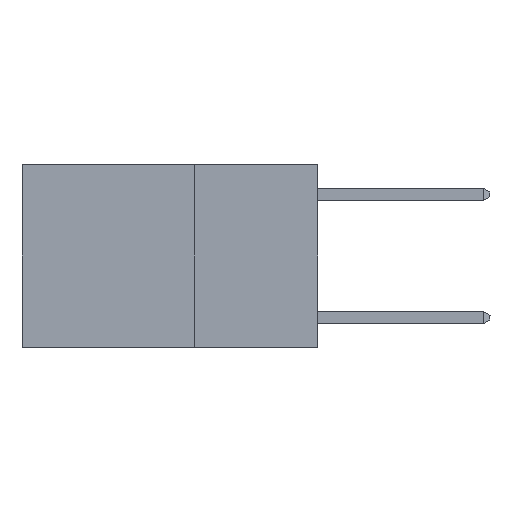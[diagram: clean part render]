
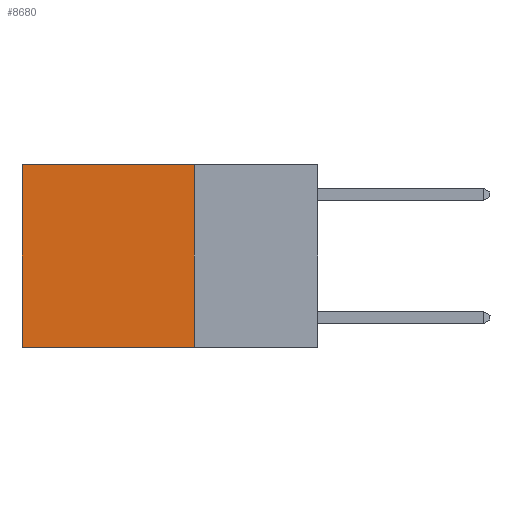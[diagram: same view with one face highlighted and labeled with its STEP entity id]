
A CAD part, left-side view. The second image highlights one B-rep face of the part: STEP entity #8680.
In plain terms, the highlighted planar face has unit normal (-1, 0, 0).
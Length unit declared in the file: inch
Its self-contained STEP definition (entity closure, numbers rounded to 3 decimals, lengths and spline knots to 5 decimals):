
#239 = LINE ( 'NONE', #921, #6667 ) ;
#490 = DIRECTION ( 'NONE',  ( 0., 0., -1. ) ) ;
#635 = AXIS2_PLACEMENT_3D ( 'NONE', #1219, #5118, #490 ) ;
#921 = CARTESIAN_POINT ( 'NONE',  ( 0.2625, 0.25, -0.37 ) ) ;
#1219 = CARTESIAN_POINT ( 'NONE',  ( 0.2625, 0.25, 0. ) ) ;
#1326 = DIRECTION ( 'NONE',  ( 0., 0., -1. ) ) ;
#1736 = CARTESIAN_POINT ( 'NONE',  ( 0.2625, 0.25, 0. ) ) ;
#1995 = VECTOR ( 'NONE', #2554, 39.37008 ) ;
#2554 = DIRECTION ( 'NONE',  ( 0., 1., 0. ) ) ;
#2725 = CARTESIAN_POINT ( 'NONE',  ( 0.2625, 0.6, -0.37 ) ) ;
#2731 = ORIENTED_EDGE ( 'NONE', *, *, #4891, .T. ) ;
#3214 = DIRECTION ( 'NONE',  ( 0., 1., 0. ) ) ;
#3255 = FACE_OUTER_BOUND ( 'NONE', #6385, .T. ) ;
#3660 = CARTESIAN_POINT ( 'NONE',  ( 0.2625, 0.6, 0. ) ) ;
#3685 = ORIENTED_EDGE ( 'NONE', *, *, #4650, .T. ) ;
#4029 = LINE ( 'NONE', #1736, #1995 ) ;
#4072 = CARTESIAN_POINT ( 'NONE',  ( 0.2625, 0.25, 0. ) ) ;
#4367 = VECTOR ( 'NONE', #1326, 39.37008 ) ;
#4582 = DIRECTION ( 'NONE',  ( 0., 0., -1. ) ) ;
#4650 = EDGE_CURVE ( 'NONE', #6990, #9124, #8582, .T. ) ;
#4891 = EDGE_CURVE ( 'NONE', #4920, #6990, #4029, .T. ) ;
#4920 = VERTEX_POINT ( 'NONE', #4072 ) ;
#5118 = DIRECTION ( 'NONE',  ( 1., 0., 0. ) ) ;
#5202 = CARTESIAN_POINT ( 'NONE',  ( 0.2625, 0.25, 0. ) ) ;
#6366 = EDGE_CURVE ( 'NONE', #4920, #9557, #6687, .T. ) ;
#6385 = EDGE_LOOP ( 'NONE', ( #3685, #6828, #8260, #2731 ) ) ;
#6483 = VECTOR ( 'NONE', #4582, 39.37008 ) ;
#6667 = VECTOR ( 'NONE', #3214, 39.37008 ) ;
#6687 = LINE ( 'NONE', #5202, #4367 ) ;
#6828 = ORIENTED_EDGE ( 'NONE', *, *, #7225, .F. ) ;
#6990 = VERTEX_POINT ( 'NONE', #3660 ) ;
#7225 = EDGE_CURVE ( 'NONE', #9557, #9124, #239, .T. ) ;
#8260 = ORIENTED_EDGE ( 'NONE', *, *, #6366, .F. ) ;
#8267 = CARTESIAN_POINT ( 'NONE',  ( 0.2625, 0.6, 0. ) ) ;
#8582 = LINE ( 'NONE', #8267, #6483 ) ;
#8680 = ADVANCED_FACE ( 'NONE', ( #3255 ), #9405, .F. ) ;
#9040 = CARTESIAN_POINT ( 'NONE',  ( 0.2625, 0.25, -0.37 ) ) ;
#9124 = VERTEX_POINT ( 'NONE', #2725 ) ;
#9405 = PLANE ( 'NONE',  #635 ) ;
#9557 = VERTEX_POINT ( 'NONE', #9040 ) ;
